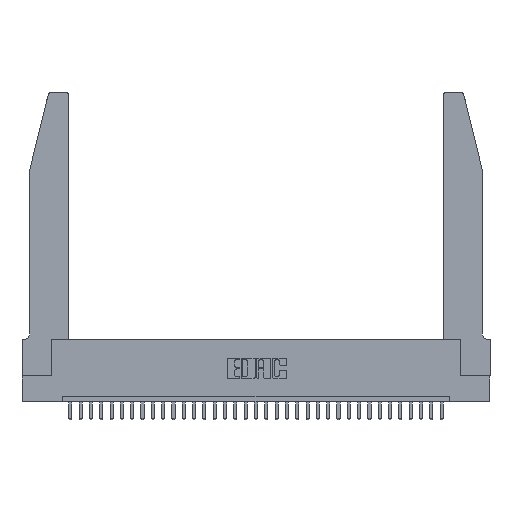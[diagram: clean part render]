
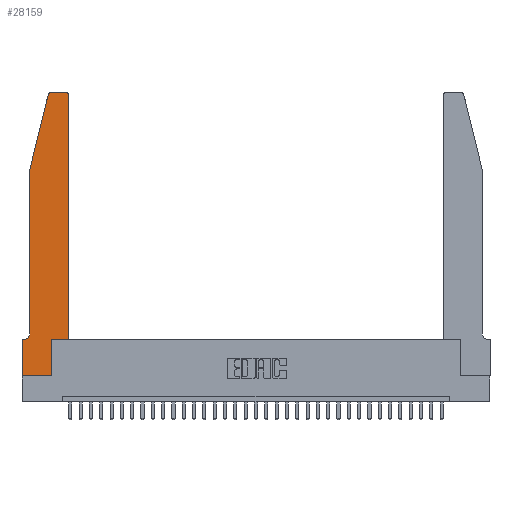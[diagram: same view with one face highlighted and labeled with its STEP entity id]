
A CAD part, top view. The second image highlights one B-rep face of the part: STEP entity #28159.
In plain terms, the highlighted planar face has unit normal (0, 0, 1).
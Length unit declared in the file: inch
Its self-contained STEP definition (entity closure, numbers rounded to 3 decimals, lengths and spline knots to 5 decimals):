
#53 = EDGE_CURVE ( 'NONE', #11391, #12133, #14413, .T. ) ;
#1311 = CARTESIAN_POINT ( 'NONE',  ( 0.4505, 0.35, 0.37 ) ) ;
#1346 = ORIENTED_EDGE ( 'NONE', *, *, #32872, .T. ) ;
#1378 = CARTESIAN_POINT ( 'NONE',  ( 0.284, 2.72, 0.37 ) ) ;
#1426 = ORIENTED_EDGE ( 'NONE', *, *, #12829, .T. ) ;
#1699 = VERTEX_POINT ( 'NONE', #12876 ) ;
#2806 = DIRECTION ( 'NONE',  ( 0., 0., 1. ) ) ;
#3082 = CARTESIAN_POINT ( 'NONE',  ( 0., 0., 0.37 ) ) ;
#3397 = CARTESIAN_POINT ( 'NONE',  ( 0.284, 2.75, 0.37 ) ) ;
#3494 = AXIS2_PLACEMENT_3D ( 'NONE', #1378, #19072, #14260 ) ;
#3658 = CARTESIAN_POINT ( 'NONE',  ( 0., 0., 0.37 ) ) ;
#4049 = CARTESIAN_POINT ( 'NONE',  ( 0.2865, 0.35, 0.37 ) ) ;
#4072 = VERTEX_POINT ( 'NONE', #6399 ) ;
#4089 = EDGE_CURVE ( 'NONE', #12841, #1699, #27613, .T. ) ;
#4159 = DIRECTION ( 'NONE',  ( 0., 1., 0. ) ) ;
#5016 = LINE ( 'NONE', #3658, #17035 ) ;
#5313 = EDGE_CURVE ( 'NONE', #22984, #16342, #31137, .T. ) ;
#6067 = PLANE ( 'NONE',  #16078 ) ;
#6377 = LINE ( 'NONE', #19294, #23264 ) ;
#6399 = CARTESIAN_POINT ( 'NONE',  ( 0.2865, 0., 0.37 ) ) ;
#6482 = CARTESIAN_POINT ( 'NONE',  ( 0.4205, 2.72, 0.37 ) ) ;
#7403 = LINE ( 'NONE', #15617, #13429 ) ;
#7538 = CARTESIAN_POINT ( 'NONE',  ( 0.0755, 2., 0.37 ) ) ;
#8118 = ORIENTED_EDGE ( 'NONE', *, *, #22437, .T. ) ;
#8236 = FACE_OUTER_BOUND ( 'NONE', #31301, .T. ) ;
#9053 = LINE ( 'NONE', #22791, #28778 ) ;
#10104 = AXIS2_PLACEMENT_3D ( 'NONE', #30935, #10128, #15609 ) ;
#10126 = DIRECTION ( 'NONE',  ( 0., 1., 0. ) ) ;
#10127 = ORIENTED_EDGE ( 'NONE', *, *, #10682, .T. ) ;
#10128 = DIRECTION ( 'NONE',  ( 0., 0., -1. ) ) ;
#10682 = EDGE_CURVE ( 'NONE', #28297, #32256, #7403, .T. ) ;
#11335 = CARTESIAN_POINT ( 'NONE',  ( 0.2865, 0.35, 0.37 ) ) ;
#11391 = VERTEX_POINT ( 'NONE', #19481 ) ;
#12133 = VERTEX_POINT ( 'NONE', #16152 ) ;
#12699 = ORIENTED_EDGE ( 'NONE', *, *, #30036, .T. ) ;
#12730 = CIRCLE ( 'NONE', #18509, 0.03 ) ;
#12829 = EDGE_CURVE ( 'NONE', #1699, #22984, #12730, .T. ) ;
#12841 = VERTEX_POINT ( 'NONE', #1311 ) ;
#12876 = CARTESIAN_POINT ( 'NONE',  ( 0.4505, 2.72, 0.37 ) ) ;
#13429 = VECTOR ( 'NONE', #23501, 39.37008 ) ;
#14260 = DIRECTION ( 'NONE',  ( 1., 0., 0. ) ) ;
#14413 = CIRCLE ( 'NONE', #10104, 0.07 ) ;
#14673 = EDGE_CURVE ( 'NONE', #16342, #28297, #20253, .T. ) ;
#14926 = LINE ( 'NONE', #21739, #20136 ) ;
#15609 = DIRECTION ( 'NONE',  ( -1., 0., 0. ) ) ;
#15617 = CARTESIAN_POINT ( 'NONE',  ( 0.0755, 2., 0.37 ) ) ;
#15717 = EDGE_CURVE ( 'NONE', #12133, #27052, #14926, .T. ) ;
#16078 = AXIS2_PLACEMENT_3D ( 'NONE', #18258, #2806, #18824 ) ;
#16152 = CARTESIAN_POINT ( 'NONE',  ( 0.0055, 0.35, 0.37 ) ) ;
#16213 = DIRECTION ( 'NONE',  ( -1., 0., 0. ) ) ;
#16342 = VERTEX_POINT ( 'NONE', #3397 ) ;
#16868 = CARTESIAN_POINT ( 'NONE',  ( 0., 0., 0.37 ) ) ;
#17035 = VECTOR ( 'NONE', #31552, 39.37008 ) ;
#17199 = DIRECTION ( 'NONE',  ( 1., 0., 0. ) ) ;
#17439 = DIRECTION ( 'NONE',  ( 1., 0., 0. ) ) ;
#17538 = ORIENTED_EDGE ( 'NONE', *, *, #27282, .T. ) ;
#17912 = VECTOR ( 'NONE', #10126, 39.37008 ) ;
#18095 = ORIENTED_EDGE ( 'NONE', *, *, #23578, .T. ) ;
#18258 = CARTESIAN_POINT ( 'NONE',  ( 0., 0.35, 0.37 ) ) ;
#18509 = AXIS2_PLACEMENT_3D ( 'NONE', #6482, #27070, #17439 ) ;
#18808 = LINE ( 'NONE', #16868, #22083 ) ;
#18824 = DIRECTION ( 'NONE',  ( 1., 0., 0. ) ) ;
#19072 = DIRECTION ( 'NONE',  ( 0., 0., 1. ) ) ;
#19100 = ORIENTED_EDGE ( 'NONE', *, *, #5313, .T. ) ;
#19264 = CARTESIAN_POINT ( 'NONE',  ( 0.25487, 2.72718, 0.37 ) ) ;
#19294 = CARTESIAN_POINT ( 'NONE',  ( 0.0755, 2., 0.37 ) ) ;
#19481 = CARTESIAN_POINT ( 'NONE',  ( 0.0755, 0.42, 0.37 ) ) ;
#20136 = VECTOR ( 'NONE', #16213, 39.37008 ) ;
#20253 = CIRCLE ( 'NONE', #3494, 0.03 ) ;
#21593 = ORIENTED_EDGE ( 'NONE', *, *, #14673, .T. ) ;
#21739 = CARTESIAN_POINT ( 'NONE',  ( 0.0755, 0.35, 0.37 ) ) ;
#22083 = VECTOR ( 'NONE', #17199, 39.37008 ) ;
#22437 = EDGE_CURVE ( 'NONE', #4072, #24340, #30069, .T. ) ;
#22605 = ORIENTED_EDGE ( 'NONE', *, *, #53, .T. ) ;
#22791 = CARTESIAN_POINT ( 'NONE',  ( 0.4505, 0.35, 0.37 ) ) ;
#22984 = VERTEX_POINT ( 'NONE', #30200 ) ;
#23241 = VERTEX_POINT ( 'NONE', #3082 ) ;
#23264 = VECTOR ( 'NONE', #27017, 39.37008 ) ;
#23286 = CARTESIAN_POINT ( 'NONE',  ( 0.2605, 2.75, 0.37 ) ) ;
#23501 = DIRECTION ( 'NONE',  ( -0.239, -0.971, 0. ) ) ;
#23578 = EDGE_CURVE ( 'NONE', #27052, #23241, #5016, .T. ) ;
#24340 = VERTEX_POINT ( 'NONE', #11335 ) ;
#25212 = VECTOR ( 'NONE', #4159, 39.37008 ) ;
#26015 = DIRECTION ( 'NONE',  ( -1., 0., 0. ) ) ;
#26040 = CARTESIAN_POINT ( 'NONE',  ( 0., 0.35, 0.37 ) ) ;
#26660 = ORIENTED_EDGE ( 'NONE', *, *, #15717, .T. ) ;
#27017 = DIRECTION ( 'NONE',  ( 0., -1., 0. ) ) ;
#27052 = VERTEX_POINT ( 'NONE', #26040 ) ;
#27070 = DIRECTION ( 'NONE',  ( 0., 0., 1. ) ) ;
#27282 = EDGE_CURVE ( 'NONE', #23241, #4072, #18808, .T. ) ;
#27613 = LINE ( 'NONE', #31803, #17912 ) ;
#28159 = ADVANCED_FACE ( 'NONE', ( #8236 ), #6067, .T. ) ;
#28297 = VERTEX_POINT ( 'NONE', #19264 ) ;
#28309 = VECTOR ( 'NONE', #26015, 39.37008 ) ;
#28743 = ORIENTED_EDGE ( 'NONE', *, *, #4089, .T. ) ;
#28778 = VECTOR ( 'NONE', #30791, 39.37008 ) ;
#30036 = EDGE_CURVE ( 'NONE', #32256, #11391, #6377, .T. ) ;
#30069 = LINE ( 'NONE', #4049, #25212 ) ;
#30200 = CARTESIAN_POINT ( 'NONE',  ( 0.4205, 2.75, 0.37 ) ) ;
#30791 = DIRECTION ( 'NONE',  ( 1., 0., 0. ) ) ;
#30935 = CARTESIAN_POINT ( 'NONE',  ( 0.0055, 0.42, 0.37 ) ) ;
#31137 = LINE ( 'NONE', #23286, #28309 ) ;
#31301 = EDGE_LOOP ( 'NONE', ( #19100, #21593, #10127, #12699, #22605, #26660, #18095, #17538, #8118, #1346, #28743, #1426 ) ) ;
#31552 = DIRECTION ( 'NONE',  ( 0., -1., 0. ) ) ;
#31803 = CARTESIAN_POINT ( 'NONE',  ( 0.4505, 0.35, 0.37 ) ) ;
#32256 = VERTEX_POINT ( 'NONE', #7538 ) ;
#32872 = EDGE_CURVE ( 'NONE', #24340, #12841, #9053, .T. ) ;
